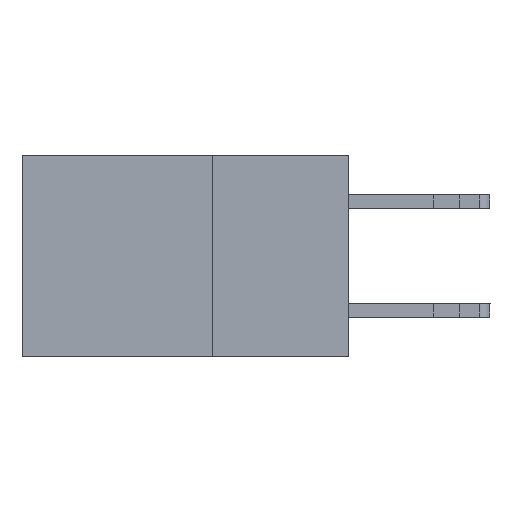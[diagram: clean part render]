
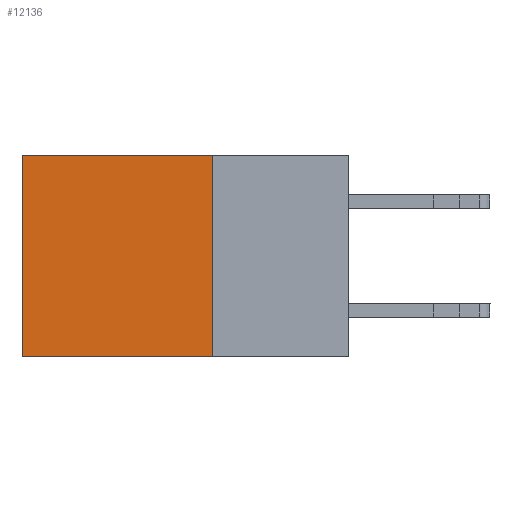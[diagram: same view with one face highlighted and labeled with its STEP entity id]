
A CAD part, left-side view. The second image highlights one B-rep face of the part: STEP entity #12136.
In plain terms, the highlighted planar face has unit normal (-1, 0, 0).
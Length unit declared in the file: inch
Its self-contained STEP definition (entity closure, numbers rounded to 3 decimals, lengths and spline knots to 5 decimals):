
#267 = DIRECTION ( 'NONE',  ( 0., 1., 0. ) ) ;
#699 = DIRECTION ( 'NONE',  ( 0., 0., -1. ) ) ;
#1219 = DIRECTION ( 'NONE',  ( 1., 0., 0. ) ) ;
#2198 = CARTESIAN_POINT ( 'NONE',  ( 0.298, 0.6, 0. ) ) ;
#2347 = VECTOR ( 'NONE', #12513, 39.37008 ) ;
#3027 = VECTOR ( 'NONE', #17460, 39.37008 ) ;
#4748 = VECTOR ( 'NONE', #699, 39.37008 ) ;
#5171 = VERTEX_POINT ( 'NONE', #5980 ) ;
#5575 = LINE ( 'NONE', #17003, #9911 ) ;
#5980 = CARTESIAN_POINT ( 'NONE',  ( 0.298, 0.6, -0.37 ) ) ;
#6252 = EDGE_LOOP ( 'NONE', ( #9889, #8923, #10435, #9076 ) ) ;
#6429 = EDGE_CURVE ( 'NONE', #16226, #6585, #15383, .T. ) ;
#6585 = VERTEX_POINT ( 'NONE', #7120 ) ;
#7120 = CARTESIAN_POINT ( 'NONE',  ( 0.298, 0.25, -0.37 ) ) ;
#7671 = LINE ( 'NONE', #7764, #3027 ) ;
#7764 = CARTESIAN_POINT ( 'NONE',  ( 0.298, 0.25, 0. ) ) ;
#8780 = FACE_OUTER_BOUND ( 'NONE', #6252, .T. ) ;
#8923 = ORIENTED_EDGE ( 'NONE', *, *, #9987, .F. ) ;
#9014 = EDGE_CURVE ( 'NONE', #17677, #5171, #11323, .T. ) ;
#9076 = ORIENTED_EDGE ( 'NONE', *, *, #16815, .T. ) ;
#9889 = ORIENTED_EDGE ( 'NONE', *, *, #9014, .T. ) ;
#9911 = VECTOR ( 'NONE', #267, 39.37008 ) ;
#9987 = EDGE_CURVE ( 'NONE', #6585, #5171, #5575, .T. ) ;
#10435 = ORIENTED_EDGE ( 'NONE', *, *, #6429, .F. ) ;
#10575 = CARTESIAN_POINT ( 'NONE',  ( 0.298, 0.6, 0. ) ) ;
#11323 = LINE ( 'NONE', #10575, #4748 ) ;
#12136 = ADVANCED_FACE ( 'NONE', ( #8780 ), #12386, .F. ) ;
#12386 = PLANE ( 'NONE',  #17069 ) ;
#12513 = DIRECTION ( 'NONE',  ( 0., 0., -1. ) ) ;
#14040 = DIRECTION ( 'NONE',  ( 0., 0., -1. ) ) ;
#15383 = LINE ( 'NONE', #15877, #2347 ) ;
#15877 = CARTESIAN_POINT ( 'NONE',  ( 0.298, 0.25, 0. ) ) ;
#16212 = CARTESIAN_POINT ( 'NONE',  ( 0.298, 0.25, 0. ) ) ;
#16226 = VERTEX_POINT ( 'NONE', #16212 ) ;
#16815 = EDGE_CURVE ( 'NONE', #16226, #17677, #7671, .T. ) ;
#17003 = CARTESIAN_POINT ( 'NONE',  ( 0.298, 0.25, -0.37 ) ) ;
#17069 = AXIS2_PLACEMENT_3D ( 'NONE', #17917, #1219, #14040 ) ;
#17460 = DIRECTION ( 'NONE',  ( 0., 1., 0. ) ) ;
#17677 = VERTEX_POINT ( 'NONE', #2198 ) ;
#17917 = CARTESIAN_POINT ( 'NONE',  ( 0.298, 0.25, 0. ) ) ;
